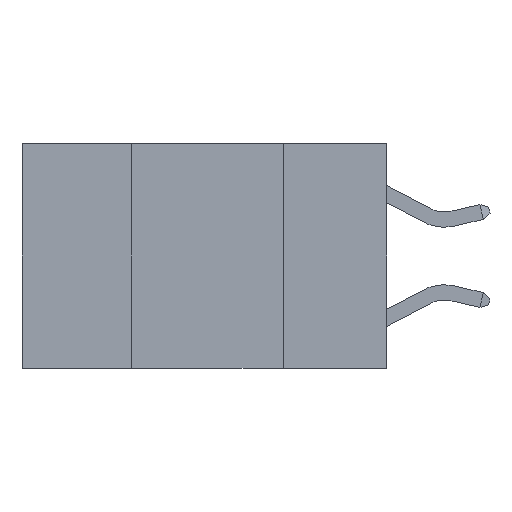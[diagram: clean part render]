
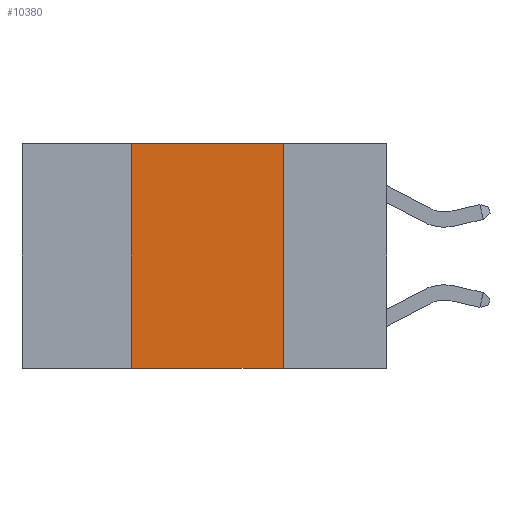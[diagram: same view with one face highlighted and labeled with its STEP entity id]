
A CAD part, left-side view. The second image highlights one B-rep face of the part: STEP entity #10380.
In plain terms, the highlighted planar face has unit normal (-1, 0, 0).
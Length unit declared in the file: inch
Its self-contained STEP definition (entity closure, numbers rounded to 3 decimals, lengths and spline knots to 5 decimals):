
#16 = EDGE_LOOP ( 'NONE', ( #5868, #3456, #8886, #6500 ) ) ;
#91 = DIRECTION ( 'NONE',  ( 0., 0., 1. ) ) ;
#216 = VERTEX_POINT ( 'NONE', #5299 ) ;
#373 = VECTOR ( 'NONE', #11608, 39.37008 ) ;
#2501 = CARTESIAN_POINT ( 'NONE',  ( 0., 0.6, -0.37 ) ) ;
#2673 = EDGE_CURVE ( 'NONE', #4666, #216, #12347, .T. ) ;
#2695 = VERTEX_POINT ( 'NONE', #9282 ) ;
#3125 = DIRECTION ( 'NONE',  ( 0., 0., -1. ) ) ;
#3144 = DIRECTION ( 'NONE',  ( 0., -1., 0. ) ) ;
#3450 = VECTOR ( 'NONE', #3125, 39.37008 ) ;
#3456 = ORIENTED_EDGE ( 'NONE', *, *, #2673, .F. ) ;
#3751 = DIRECTION ( 'NONE',  ( 0., 0., -1. ) ) ;
#3794 = LINE ( 'NONE', #10229, #8903 ) ;
#4516 = AXIS2_PLACEMENT_3D ( 'NONE', #8843, #9877, #3751 ) ;
#4666 = VERTEX_POINT ( 'NONE', #9520 ) ;
#4742 = EDGE_CURVE ( 'NONE', #2695, #13143, #11508, .T. ) ;
#4744 = PLANE ( 'NONE',  #4516 ) ;
#5299 = CARTESIAN_POINT ( 'NONE',  ( 0., 0.17, 0. ) ) ;
#5580 = CARTESIAN_POINT ( 'NONE',  ( 0., 0.17, -0.37 ) ) ;
#5868 = ORIENTED_EDGE ( 'NONE', *, *, #12906, .F. ) ;
#6108 = EDGE_CURVE ( 'NONE', #2695, #4666, #3794, .T. ) ;
#6197 = CARTESIAN_POINT ( 'NONE',  ( 0., 0.17, 0. ) ) ;
#6500 = ORIENTED_EDGE ( 'NONE', *, *, #4742, .T. ) ;
#8806 = FACE_OUTER_BOUND ( 'NONE', #16, .T. ) ;
#8843 = CARTESIAN_POINT ( 'NONE',  ( 0., 0.6, 0. ) ) ;
#8878 = LINE ( 'NONE', #6197, #3450 ) ;
#8886 = ORIENTED_EDGE ( 'NONE', *, *, #6108, .F. ) ;
#8903 = VECTOR ( 'NONE', #91, 39.37008 ) ;
#9282 = CARTESIAN_POINT ( 'NONE',  ( 0., 0.42, -0.37 ) ) ;
#9520 = CARTESIAN_POINT ( 'NONE',  ( 0., 0.42, 0. ) ) ;
#9652 = VECTOR ( 'NONE', #3144, 39.37008 ) ;
#9877 = DIRECTION ( 'NONE',  ( 1., 0., 0. ) ) ;
#10229 = CARTESIAN_POINT ( 'NONE',  ( 0., 0.42, 0. ) ) ;
#10380 = ADVANCED_FACE ( 'NONE', ( #8806 ), #4744, .F. ) ;
#10573 = CARTESIAN_POINT ( 'NONE',  ( 0., 0.6, 0. ) ) ;
#11508 = LINE ( 'NONE', #2501, #373 ) ;
#11608 = DIRECTION ( 'NONE',  ( 0., -1., 0. ) ) ;
#12347 = LINE ( 'NONE', #10573, #9652 ) ;
#12906 = EDGE_CURVE ( 'NONE', #216, #13143, #8878, .T. ) ;
#13143 = VERTEX_POINT ( 'NONE', #5580 ) ;
